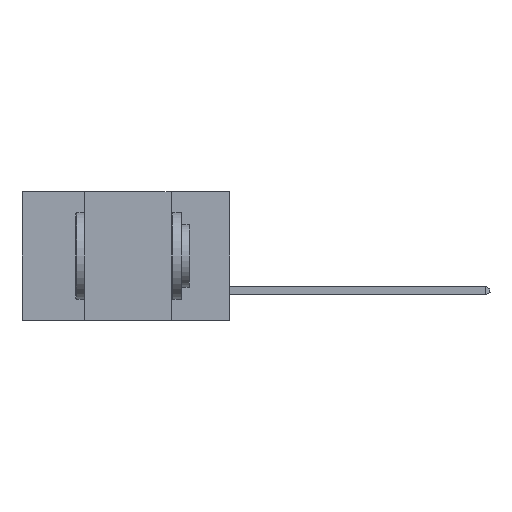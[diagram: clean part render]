
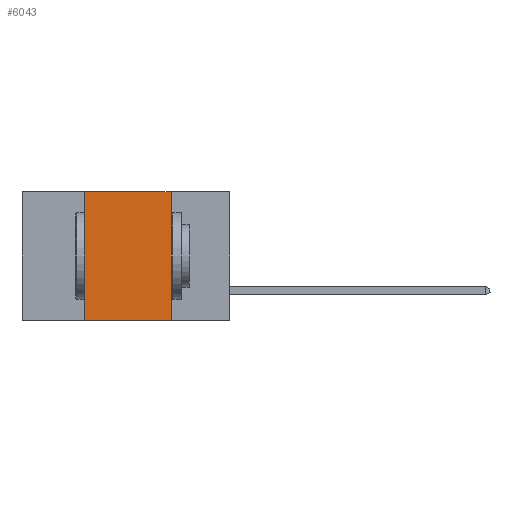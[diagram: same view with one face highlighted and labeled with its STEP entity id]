
A CAD part, left-side view. The second image highlights one B-rep face of the part: STEP entity #6043.
In plain terms, the highlighted planar face has unit normal (-1, 0, 0).
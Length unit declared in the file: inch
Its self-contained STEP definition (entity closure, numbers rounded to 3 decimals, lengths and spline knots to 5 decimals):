
#292 = ORIENTED_EDGE ( 'NONE', *, *, #8937, .F. ) ;
#409 = LINE ( 'NONE', #649, #1814 ) ;
#649 = CARTESIAN_POINT ( 'NONE',  ( 0., 0.6, -0.37 ) ) ;
#860 = DIRECTION ( 'NONE',  ( 0., 0., -1. ) ) ;
#932 = FACE_OUTER_BOUND ( 'NONE', #2253, .T. ) ;
#1488 = CARTESIAN_POINT ( 'NONE',  ( 0., 0.17, 0. ) ) ;
#1528 = ORIENTED_EDGE ( 'NONE', *, *, #8962, .T. ) ;
#1814 = VECTOR ( 'NONE', #8439, 39.37008 ) ;
#2228 = VECTOR ( 'NONE', #13436, 39.37008 ) ;
#2253 = EDGE_LOOP ( 'NONE', ( #3013, #292, #11391, #1528 ) ) ;
#3013 = ORIENTED_EDGE ( 'NONE', *, *, #5733, .F. ) ;
#3899 = CARTESIAN_POINT ( 'NONE',  ( 0., 0.42, 0. ) ) ;
#4482 = CARTESIAN_POINT ( 'NONE',  ( 0., 0.6, 0. ) ) ;
#5693 = VERTEX_POINT ( 'NONE', #15990 ) ;
#5733 = EDGE_CURVE ( 'NONE', #13913, #5693, #10019, .T. ) ;
#6043 = ADVANCED_FACE ( 'NONE', ( #932 ), #16295, .F. ) ;
#7265 = CARTESIAN_POINT ( 'NONE',  ( 0., 0.6, 0. ) ) ;
#7932 = AXIS2_PLACEMENT_3D ( 'NONE', #7265, #8621, #9913 ) ;
#8439 = DIRECTION ( 'NONE',  ( 0., -1., 0. ) ) ;
#8621 = DIRECTION ( 'NONE',  ( 1., 0., 0. ) ) ;
#8937 = EDGE_CURVE ( 'NONE', #13937, #13913, #13689, .T. ) ;
#8962 = EDGE_CURVE ( 'NONE', #9201, #5693, #409, .T. ) ;
#9201 = VERTEX_POINT ( 'NONE', #12363 ) ;
#9619 = VECTOR ( 'NONE', #860, 39.37008 ) ;
#9913 = DIRECTION ( 'NONE',  ( 0., 0., -1. ) ) ;
#10019 = LINE ( 'NONE', #12309, #9619 ) ;
#11391 = ORIENTED_EDGE ( 'NONE', *, *, #15595, .F. ) ;
#12309 = CARTESIAN_POINT ( 'NONE',  ( 0., 0.17, 0. ) ) ;
#12363 = CARTESIAN_POINT ( 'NONE',  ( 0., 0.42, -0.37 ) ) ;
#12914 = CARTESIAN_POINT ( 'NONE',  ( 0., 0.42, 0. ) ) ;
#13436 = DIRECTION ( 'NONE',  ( 0., -1., 0. ) ) ;
#13689 = LINE ( 'NONE', #4482, #2228 ) ;
#13913 = VERTEX_POINT ( 'NONE', #1488 ) ;
#13937 = VERTEX_POINT ( 'NONE', #3899 ) ;
#14376 = VECTOR ( 'NONE', #15307, 39.37008 ) ;
#15307 = DIRECTION ( 'NONE',  ( 0., 0., 1. ) ) ;
#15595 = EDGE_CURVE ( 'NONE', #9201, #13937, #16164, .T. ) ;
#15990 = CARTESIAN_POINT ( 'NONE',  ( 0., 0.17, -0.37 ) ) ;
#16164 = LINE ( 'NONE', #12914, #14376 ) ;
#16295 = PLANE ( 'NONE',  #7932 ) ;
